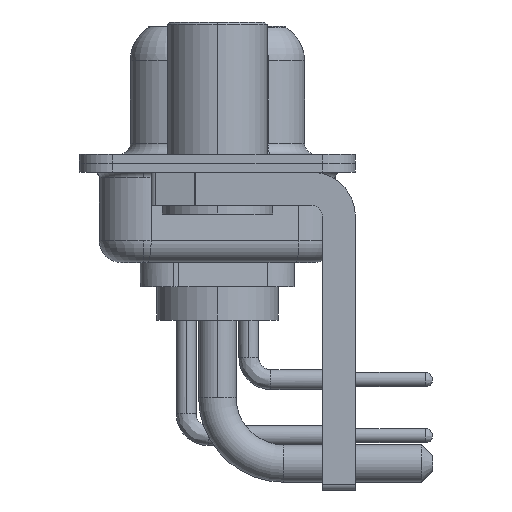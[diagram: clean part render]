
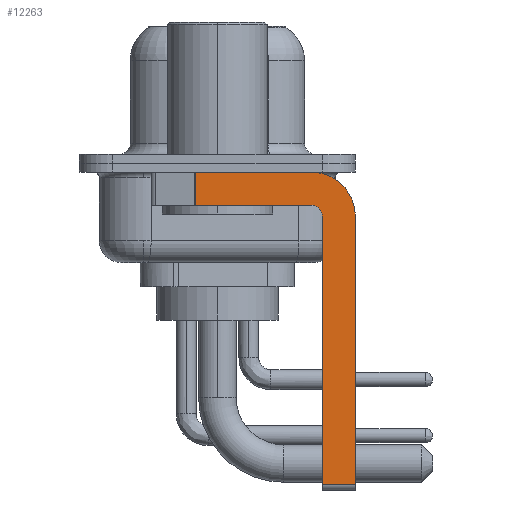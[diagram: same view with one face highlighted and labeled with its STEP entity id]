
A CAD part, left-side view. The second image highlights one B-rep face of the part: STEP entity #12263.
In plain terms, the highlighted planar face has unit normal (-1, 0, 0).
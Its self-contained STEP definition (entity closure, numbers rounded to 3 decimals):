
#35 = CARTESIAN_POINT ( 'NONE',  ( -2.9, -4.25, -14.55 ) ) ;
#393 = VERTEX_POINT ( 'NONE', #4965 ) ;
#493 = VECTOR ( 'NONE', #4696, 1000. ) ;
#734 = EDGE_CURVE ( 'NONE', #3002, #8694, #13591, .T. ) ;
#1267 = PLANE ( 'NONE',  #17766 ) ;
#1494 = CARTESIAN_POINT ( 'NONE',  ( -2.9, -4.25, -2.4 ) ) ;
#2054 = CARTESIAN_POINT ( 'NONE',  ( -2.9, -4.75, -14.55 ) ) ;
#2332 = VERTEX_POINT ( 'NONE', #2054 ) ;
#2927 = DIRECTION ( 'NONE',  ( 1., 0., 0. ) ) ;
#3002 = VERTEX_POINT ( 'NONE', #20553 ) ;
#3053 = DIRECTION ( 'NONE',  ( 0., 1., 0. ) ) ;
#3118 = VERTEX_POINT ( 'NONE', #14896 ) ;
#3798 = LINE ( 'NONE', #3915, #22378 ) ;
#3915 = CARTESIAN_POINT ( 'NONE',  ( -2.9, -6.25, -2.4 ) ) ;
#4441 = VERTEX_POINT ( 'NONE', #10767 ) ;
#4696 = DIRECTION ( 'NONE',  ( 0., -1., 0. ) ) ;
#4764 = VECTOR ( 'NONE', #23262, 1000. ) ;
#4961 = EDGE_CURVE ( 'NONE', #2332, #4441, #6967, .T. ) ;
#4965 = CARTESIAN_POINT ( 'NONE',  ( -2.9, -6.25, -14.55 ) ) ;
#5162 = VECTOR ( 'NONE', #19997, 1000. ) ;
#5270 = DIRECTION ( 'NONE',  ( 1., 0., 0. ) ) ;
#5922 = CIRCLE ( 'NONE', #15745, 0.5 ) ;
#6304 = EDGE_CURVE ( 'NONE', #8694, #3118, #12760, .T. ) ;
#6480 = CARTESIAN_POINT ( 'NONE',  ( -2.9, -4.25, -2.4 ) ) ;
#6739 = CARTESIAN_POINT ( 'NONE',  ( -2.9, -4.25, -1.9 ) ) ;
#6936 = EDGE_CURVE ( 'NONE', #2332, #393, #16233, .T. ) ;
#6967 = LINE ( 'NONE', #14185, #4764 ) ;
#6969 = CARTESIAN_POINT ( 'NONE',  ( -2.9, -4.25, -2.4 ) ) ;
#7037 = VERTEX_POINT ( 'NONE', #13634 ) ;
#8136 = LINE ( 'NONE', #18758, #15299 ) ;
#8694 = VERTEX_POINT ( 'NONE', #13083 ) ;
#10025 = DIRECTION ( 'NONE',  ( 0., 0., -1. ) ) ;
#10148 = EDGE_CURVE ( 'NONE', #7037, #13953, #17467, .T. ) ;
#10171 = EDGE_LOOP ( 'NONE', ( #14098, #16313, #18007, #17214, #13003, #19973, #20147, #12086 ) ) ;
#10486 = DIRECTION ( 'NONE',  ( 0., 0., -1. ) ) ;
#10767 = CARTESIAN_POINT ( 'NONE',  ( -2.9, -4.75, -2.4 ) ) ;
#12086 = ORIENTED_EDGE ( 'NONE', *, *, #6304, .F. ) ;
#12263 = ADVANCED_FACE ( 'NONE', ( #21128 ), #1267, .F. ) ;
#12760 = CIRCLE ( 'NONE', #17969, 2. ) ;
#13003 = ORIENTED_EDGE ( 'NONE', *, *, #4961, .F. ) ;
#13083 = CARTESIAN_POINT ( 'NONE',  ( -2.9, -4.25, -0.4 ) ) ;
#13591 = LINE ( 'NONE', #20774, #493 ) ;
#13634 = CARTESIAN_POINT ( 'NONE',  ( -2.9, -4.25, -1.9 ) ) ;
#13719 = DIRECTION ( 'NONE',  ( 0., 0., 1. ) ) ;
#13953 = VERTEX_POINT ( 'NONE', #19289 ) ;
#14098 = ORIENTED_EDGE ( 'NONE', *, *, #734, .F. ) ;
#14185 = CARTESIAN_POINT ( 'NONE',  ( -2.9, -4.75, -14.8 ) ) ;
#14896 = CARTESIAN_POINT ( 'NONE',  ( -2.9, -6.25, -2.4 ) ) ;
#15099 = VECTOR ( 'NONE', #3053, 1000. ) ;
#15299 = VECTOR ( 'NONE', #20772, 1000. ) ;
#15745 = AXIS2_PLACEMENT_3D ( 'NONE', #6969, #20903, #13719 ) ;
#16233 = LINE ( 'NONE', #35, #5162 ) ;
#16313 = ORIENTED_EDGE ( 'NONE', *, *, #19476, .T. ) ;
#17214 = ORIENTED_EDGE ( 'NONE', *, *, #22241, .F. ) ;
#17449 = EDGE_CURVE ( 'NONE', #3118, #393, #3798, .T. ) ;
#17467 = LINE ( 'NONE', #6739, #15099 ) ;
#17766 = AXIS2_PLACEMENT_3D ( 'NONE', #6480, #2927, #10025 ) ;
#17969 = AXIS2_PLACEMENT_3D ( 'NONE', #1494, #5270, #10486 ) ;
#18007 = ORIENTED_EDGE ( 'NONE', *, *, #10148, .F. ) ;
#18314 = DIRECTION ( 'NONE',  ( 0., 0., -1. ) ) ;
#18758 = CARTESIAN_POINT ( 'NONE',  ( -2.9, 0.978, -1.9 ) ) ;
#19289 = CARTESIAN_POINT ( 'NONE',  ( -2.9, 0.978, -1.9 ) ) ;
#19476 = EDGE_CURVE ( 'NONE', #3002, #13953, #8136, .T. ) ;
#19973 = ORIENTED_EDGE ( 'NONE', *, *, #6936, .T. ) ;
#19997 = DIRECTION ( 'NONE',  ( 0., -1., 0. ) ) ;
#20147 = ORIENTED_EDGE ( 'NONE', *, *, #17449, .F. ) ;
#20553 = CARTESIAN_POINT ( 'NONE',  ( -2.9, 0.978, -0.4 ) ) ;
#20772 = DIRECTION ( 'NONE',  ( 0., 0., -1. ) ) ;
#20774 = CARTESIAN_POINT ( 'NONE',  ( -2.9, 3., -0.4 ) ) ;
#20903 = DIRECTION ( 'NONE',  ( -1., 0., 0. ) ) ;
#21128 = FACE_OUTER_BOUND ( 'NONE', #10171, .T. ) ;
#22241 = EDGE_CURVE ( 'NONE', #4441, #7037, #5922, .T. ) ;
#22378 = VECTOR ( 'NONE', #18314, 1000. ) ;
#23262 = DIRECTION ( 'NONE',  ( 0., 0., 1. ) ) ;
